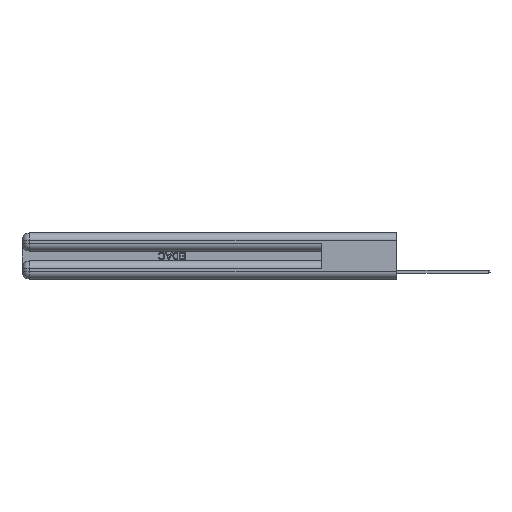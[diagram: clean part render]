
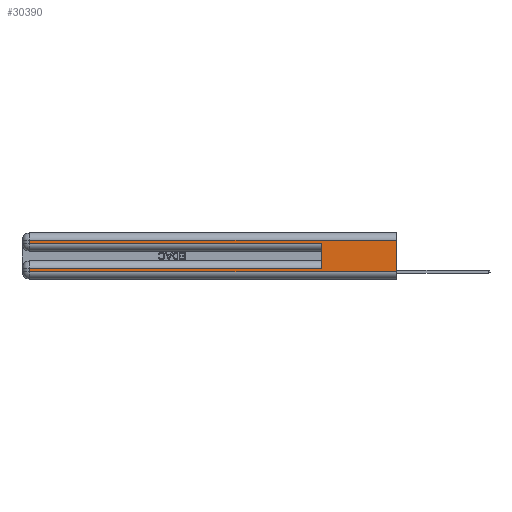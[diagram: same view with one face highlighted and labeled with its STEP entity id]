
A CAD part, left-side view. The second image highlights one B-rep face of the part: STEP entity #30390.
In plain terms, the highlighted planar face has unit normal (-1, 0, 0).
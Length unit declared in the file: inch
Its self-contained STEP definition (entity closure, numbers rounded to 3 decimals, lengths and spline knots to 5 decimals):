
#324 = DIRECTION ( 'NONE',  ( 0., -1., 0. ) ) ;
#1320 = DIRECTION ( 'NONE',  ( 0., 0., -1. ) ) ;
#3539 = DIRECTION ( 'NONE',  ( 0., 0., 1. ) ) ;
#3769 = CARTESIAN_POINT ( 'NONE',  ( 0., 0.6, 0.145 ) ) ;
#3873 = CARTESIAN_POINT ( 'NONE',  ( 0., 2.94, 0.085 ) ) ;
#3926 = VECTOR ( 'NONE', #15190, 39.37008 ) ;
#4738 = LINE ( 'NONE', #15077, #3926 ) ;
#5157 = VERTEX_POINT ( 'NONE', #21321 ) ;
#6000 = LINE ( 'NONE', #3769, #13164 ) ;
#6030 = VECTOR ( 'NONE', #20034, 39.37008 ) ;
#6568 = EDGE_CURVE ( 'NONE', #8514, #25961, #21702, .T. ) ;
#8235 = CARTESIAN_POINT ( 'NONE',  ( 0., 0., 0.37 ) ) ;
#8514 = VERTEX_POINT ( 'NONE', #3873 ) ;
#8671 = CARTESIAN_POINT ( 'NONE',  ( 0., 2.94, 0.37 ) ) ;
#8772 = DIRECTION ( 'NONE',  ( 0., 0., -1. ) ) ;
#9030 = CARTESIAN_POINT ( 'NONE',  ( 0., 0., 0.37 ) ) ;
#9387 = EDGE_CURVE ( 'NONE', #16973, #5157, #28755, .T. ) ;
#9491 = EDGE_CURVE ( 'NONE', #26876, #16973, #20267, .T. ) ;
#9802 = CARTESIAN_POINT ( 'NONE',  ( 0., 0., 0.06 ) ) ;
#10251 = CARTESIAN_POINT ( 'NONE',  ( 0., 2.94, 0.37 ) ) ;
#10581 = VECTOR ( 'NONE', #324, 39.37008 ) ;
#11033 = ORIENTED_EDGE ( 'NONE', *, *, #9491, .T. ) ;
#12012 = LINE ( 'NONE', #25028, #6030 ) ;
#12428 = CARTESIAN_POINT ( 'NONE',  ( 0., 2.94, 0.06 ) ) ;
#12821 = ORIENTED_EDGE ( 'NONE', *, *, #9387, .T. ) ;
#13164 = VECTOR ( 'NONE', #3539, 39.37008 ) ;
#13629 = VERTEX_POINT ( 'NONE', #9802 ) ;
#14852 = VECTOR ( 'NONE', #18000, 39.37008 ) ;
#15049 = ORIENTED_EDGE ( 'NONE', *, *, #25255, .T. ) ;
#15077 = CARTESIAN_POINT ( 'NONE',  ( 0., 0., 0.31 ) ) ;
#15190 = DIRECTION ( 'NONE',  ( 0., 1., 0. ) ) ;
#15260 = CARTESIAN_POINT ( 'NONE',  ( 0., 2.94, 0.31 ) ) ;
#15505 = EDGE_CURVE ( 'NONE', #24569, #8514, #12012, .T. ) ;
#16682 = DIRECTION ( 'NONE',  ( 1., 0., 0. ) ) ;
#16802 = PLANE ( 'NONE',  #22361 ) ;
#16901 = EDGE_CURVE ( 'NONE', #24569, #5157, #6000, .T. ) ;
#16973 = VERTEX_POINT ( 'NONE', #19696 ) ;
#17644 = ORIENTED_EDGE ( 'NONE', *, *, #30881, .T. ) ;
#17884 = CARTESIAN_POINT ( 'NONE',  ( 0., 0.6, 0.085 ) ) ;
#18000 = DIRECTION ( 'NONE',  ( 0., 0., -1. ) ) ;
#18170 = LINE ( 'NONE', #8235, #33147 ) ;
#18246 = DIRECTION ( 'NONE',  ( 0., 0., -1. ) ) ;
#18473 = ORIENTED_EDGE ( 'NONE', *, *, #6568, .T. ) ;
#18652 = CARTESIAN_POINT ( 'NONE',  ( 0., 0., 0.31 ) ) ;
#18894 = EDGE_CURVE ( 'NONE', #29465, #13629, #18170, .T. ) ;
#19619 = EDGE_LOOP ( 'NONE', ( #27349, #15049, #11033, #12821, #21958, #21795, #18473, #17644 ) ) ;
#19696 = CARTESIAN_POINT ( 'NONE',  ( 0., 2.94, 0.285 ) ) ;
#20034 = DIRECTION ( 'NONE',  ( 0., 1., 0. ) ) ;
#20267 = LINE ( 'NONE', #8671, #21889 ) ;
#21091 = VECTOR ( 'NONE', #33152, 39.37008 ) ;
#21321 = CARTESIAN_POINT ( 'NONE',  ( 0., 0.6, 0.285 ) ) ;
#21702 = LINE ( 'NONE', #10251, #14852 ) ;
#21795 = ORIENTED_EDGE ( 'NONE', *, *, #15505, .T. ) ;
#21889 = VECTOR ( 'NONE', #8772, 39.37008 ) ;
#21958 = ORIENTED_EDGE ( 'NONE', *, *, #16901, .F. ) ;
#22361 = AXIS2_PLACEMENT_3D ( 'NONE', #9030, #16682, #1320 ) ;
#23227 = CARTESIAN_POINT ( 'NONE',  ( 0., 0., 0.285 ) ) ;
#24569 = VERTEX_POINT ( 'NONE', #17884 ) ;
#25028 = CARTESIAN_POINT ( 'NONE',  ( 0., 0., 0.085 ) ) ;
#25255 = EDGE_CURVE ( 'NONE', #29465, #26876, #4738, .T. ) ;
#25428 = FACE_OUTER_BOUND ( 'NONE', #19619, .T. ) ;
#25961 = VERTEX_POINT ( 'NONE', #12428 ) ;
#26876 = VERTEX_POINT ( 'NONE', #15260 ) ;
#27349 = ORIENTED_EDGE ( 'NONE', *, *, #18894, .F. ) ;
#27408 = LINE ( 'NONE', #31062, #10581 ) ;
#28755 = LINE ( 'NONE', #23227, #21091 ) ;
#29465 = VERTEX_POINT ( 'NONE', #18652 ) ;
#30390 = ADVANCED_FACE ( 'NONE', ( #25428 ), #16802, .F. ) ;
#30881 = EDGE_CURVE ( 'NONE', #25961, #13629, #27408, .T. ) ;
#31062 = CARTESIAN_POINT ( 'NONE',  ( 0., 0., 0.06 ) ) ;
#33147 = VECTOR ( 'NONE', #18246, 39.37008 ) ;
#33152 = DIRECTION ( 'NONE',  ( 0., -1., 0. ) ) ;
